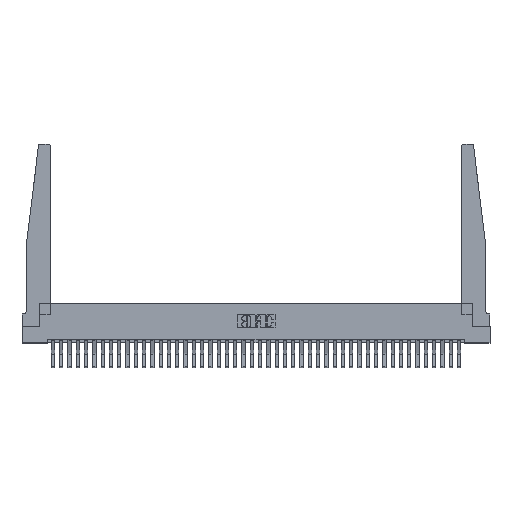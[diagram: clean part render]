
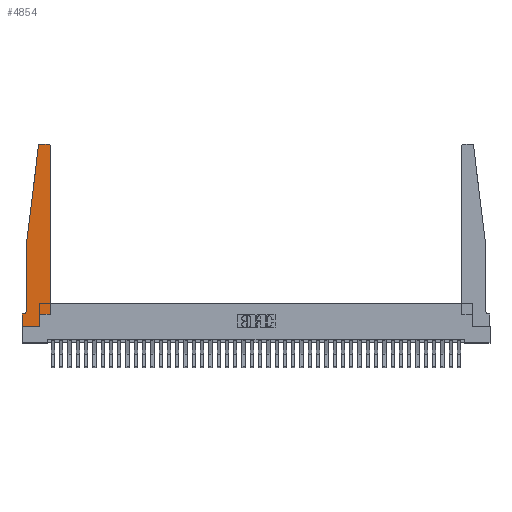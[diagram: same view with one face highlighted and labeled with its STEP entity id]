
A CAD part, top view. The second image highlights one B-rep face of the part: STEP entity #4854.
In plain terms, the highlighted planar face has unit normal (0, 0, 1).
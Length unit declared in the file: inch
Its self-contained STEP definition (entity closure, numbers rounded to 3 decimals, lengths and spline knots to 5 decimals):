
#469 = VERTEX_POINT ( 'NONE', #24913 ) ;
#730 = DIRECTION ( 'NONE',  ( 0., -1., 0. ) ) ;
#1406 = VECTOR ( 'NONE', #34349, 39.37008 ) ;
#1655 = DIRECTION ( 'NONE',  ( 0., 0., 1. ) ) ;
#2003 = EDGE_LOOP ( 'NONE', ( #2684, #4446, #31776, #13478, #16946, #12337, #13465, #21515, #30687, #9007, #33362, #3967 ) ) ;
#2256 = LINE ( 'NONE', #27699, #36144 ) ;
#2684 = ORIENTED_EDGE ( 'NONE', *, *, #27348, .T. ) ;
#2996 = VECTOR ( 'NONE', #10991, 39.37008 ) ;
#3223 = CARTESIAN_POINT ( 'NONE',  ( 0.065, 1.25, 0.37 ) ) ;
#3450 = CARTESIAN_POINT ( 'NONE',  ( 0.425, 0.18, 0.37 ) ) ;
#3483 = CARTESIAN_POINT ( 'NONE',  ( 0.425, 2.72, 0.37 ) ) ;
#3559 = VECTOR ( 'NONE', #11921, 39.37008 ) ;
#3967 = ORIENTED_EDGE ( 'NONE', *, *, #20323, .T. ) ;
#4028 = CARTESIAN_POINT ( 'NONE',  ( 0.395, 2.75, 0.37 ) ) ;
#4446 = ORIENTED_EDGE ( 'NONE', *, *, #19675, .T. ) ;
#4649 = AXIS2_PLACEMENT_3D ( 'NONE', #33127, #22322, #8237 ) ;
#4854 = ADVANCED_FACE ( 'NONE', ( #5731 ), #15746, .T. ) ;
#5681 = CARTESIAN_POINT ( 'NONE',  ( 0.2605, 0.18, 0.37 ) ) ;
#5731 = FACE_OUTER_BOUND ( 'NONE', #2003, .T. ) ;
#5926 = VERTEX_POINT ( 'NONE', #10606 ) ;
#6012 = AXIS2_PLACEMENT_3D ( 'NONE', #32309, #1655, #33043 ) ;
#6776 = VECTOR ( 'NONE', #17466, 39.37008 ) ;
#8115 = VECTOR ( 'NONE', #18488, 39.37008 ) ;
#8237 = DIRECTION ( 'NONE',  ( 1., 0., 0. ) ) ;
#8424 = CARTESIAN_POINT ( 'NONE',  ( 0.425, 0.18, 0.37 ) ) ;
#8470 = LINE ( 'NONE', #3223, #1406 ) ;
#9007 = ORIENTED_EDGE ( 'NONE', *, *, #31423, .T. ) ;
#10284 = DIRECTION ( 'NONE',  ( 1., 0., 0. ) ) ;
#10368 = DIRECTION ( 'NONE',  ( -0.122, -0.992, 0. ) ) ;
#10606 = CARTESIAN_POINT ( 'NONE',  ( 0., 0.1875, 0.37 ) ) ;
#10640 = CARTESIAN_POINT ( 'NONE',  ( 0.015, 0.1875, 0.37 ) ) ;
#10991 = DIRECTION ( 'NONE',  ( 0., 1., 0. ) ) ;
#11059 = LINE ( 'NONE', #29067, #3559 ) ;
#11267 = CIRCLE ( 'NONE', #6012, 0.03 ) ;
#11921 = DIRECTION ( 'NONE',  ( 0., 1., 0. ) ) ;
#12337 = ORIENTED_EDGE ( 'NONE', *, *, #21358, .T. ) ;
#12899 = VERTEX_POINT ( 'NONE', #5681 ) ;
#13136 = DIRECTION ( 'NONE',  ( 0., 0., 1. ) ) ;
#13337 = CARTESIAN_POINT ( 'NONE',  ( 0.065, 1.25, 0.37 ) ) ;
#13465 = ORIENTED_EDGE ( 'NONE', *, *, #36258, .T. ) ;
#13478 = ORIENTED_EDGE ( 'NONE', *, *, #14838, .T. ) ;
#14048 = CARTESIAN_POINT ( 'NONE',  ( 0.065, 0.1875, 0.37 ) ) ;
#14838 = EDGE_CURVE ( 'NONE', #36027, #19788, #8470, .T. ) ;
#15075 = LINE ( 'NONE', #13337, #19918 ) ;
#15208 = EDGE_CURVE ( 'NONE', #19788, #27316, #26507, .T. ) ;
#15484 = EDGE_CURVE ( 'NONE', #16502, #12899, #11059, .T. ) ;
#15746 = PLANE ( 'NONE',  #28295 ) ;
#16502 = VERTEX_POINT ( 'NONE', #19774 ) ;
#16516 = CARTESIAN_POINT ( 'NONE',  ( 0.015, 0.2375, 0.37 ) ) ;
#16946 = ORIENTED_EDGE ( 'NONE', *, *, #15208, .T. ) ;
#17116 = CARTESIAN_POINT ( 'NONE',  ( 0.065, 0.2375, 0.37 ) ) ;
#17466 = DIRECTION ( 'NONE',  ( -1., 0., 0. ) ) ;
#17596 = CARTESIAN_POINT ( 'NONE',  ( 0., 0., 0.37 ) ) ;
#17909 = CARTESIAN_POINT ( 'NONE',  ( 0., 0., 0.37 ) ) ;
#18488 = DIRECTION ( 'NONE',  ( 1., 0., 0. ) ) ;
#18975 = EDGE_CURVE ( 'NONE', #34360, #22185, #25064, .T. ) ;
#19044 = DIRECTION ( 'NONE',  ( -1., 0., 0. ) ) ;
#19110 = VERTEX_POINT ( 'NONE', #33644 ) ;
#19675 = EDGE_CURVE ( 'NONE', #19110, #31331, #32009, .T. ) ;
#19774 = CARTESIAN_POINT ( 'NONE',  ( 0.2605, 0., 0.37 ) ) ;
#19788 = VERTEX_POINT ( 'NONE', #17116 ) ;
#19918 = VECTOR ( 'NONE', #10368, 39.37008 ) ;
#20323 = EDGE_CURVE ( 'NONE', #22185, #35194, #11267, .T. ) ;
#20734 = VECTOR ( 'NONE', #26781, 39.37008 ) ;
#21358 = EDGE_CURVE ( 'NONE', #27316, #5926, #31042, .T. ) ;
#21515 = ORIENTED_EDGE ( 'NONE', *, *, #27843, .T. ) ;
#22185 = VERTEX_POINT ( 'NONE', #3483 ) ;
#22322 = DIRECTION ( 'NONE',  ( 0., 0., 1. ) ) ;
#24913 = CARTESIAN_POINT ( 'NONE',  ( 0., 0., 0.37 ) ) ;
#25037 = DIRECTION ( 'NONE',  ( 0., 0., -1. ) ) ;
#25064 = LINE ( 'NONE', #33419, #2996 ) ;
#26507 = CIRCLE ( 'NONE', #36132, 0.05 ) ;
#26781 = DIRECTION ( 'NONE',  ( 1., 0., 0. ) ) ;
#27316 = VERTEX_POINT ( 'NONE', #10640 ) ;
#27348 = EDGE_CURVE ( 'NONE', #35194, #19110, #2256, .T. ) ;
#27699 = CARTESIAN_POINT ( 'NONE',  ( 0.25, 2.75, 0.37 ) ) ;
#27843 = EDGE_CURVE ( 'NONE', #469, #16502, #35668, .T. ) ;
#28295 = AXIS2_PLACEMENT_3D ( 'NONE', #35500, #13136, #10284 ) ;
#28514 = CARTESIAN_POINT ( 'NONE',  ( 0.24675, 2.72367, 0.37 ) ) ;
#29067 = CARTESIAN_POINT ( 'NONE',  ( 0.2605, 0.18, 0.37 ) ) ;
#30687 = ORIENTED_EDGE ( 'NONE', *, *, #15484, .T. ) ;
#31042 = LINE ( 'NONE', #14048, #6776 ) ;
#31331 = VERTEX_POINT ( 'NONE', #28514 ) ;
#31423 = EDGE_CURVE ( 'NONE', #12899, #34360, #34109, .T. ) ;
#31776 = ORIENTED_EDGE ( 'NONE', *, *, #32940, .T. ) ;
#32009 = CIRCLE ( 'NONE', #4649, 0.03 ) ;
#32309 = CARTESIAN_POINT ( 'NONE',  ( 0.395, 2.72, 0.37 ) ) ;
#32940 = EDGE_CURVE ( 'NONE', #31331, #36027, #15075, .T. ) ;
#33043 = DIRECTION ( 'NONE',  ( 1., 0., 0. ) ) ;
#33127 = CARTESIAN_POINT ( 'NONE',  ( 0.27653, 2.72, 0.37 ) ) ;
#33246 = DIRECTION ( 'NONE',  ( -1., 0., 0. ) ) ;
#33362 = ORIENTED_EDGE ( 'NONE', *, *, #18975, .T. ) ;
#33419 = CARTESIAN_POINT ( 'NONE',  ( 0.425, 0.18, 0.37 ) ) ;
#33644 = CARTESIAN_POINT ( 'NONE',  ( 0.27653, 2.75, 0.37 ) ) ;
#34109 = LINE ( 'NONE', #3450, #8115 ) ;
#34186 = LINE ( 'NONE', #17596, #35958 ) ;
#34349 = DIRECTION ( 'NONE',  ( 0., -1., 0. ) ) ;
#34360 = VERTEX_POINT ( 'NONE', #8424 ) ;
#35194 = VERTEX_POINT ( 'NONE', #4028 ) ;
#35500 = CARTESIAN_POINT ( 'NONE',  ( 0., 0.1875, 0.37 ) ) ;
#35668 = LINE ( 'NONE', #17909, #20734 ) ;
#35681 = CARTESIAN_POINT ( 'NONE',  ( 0.065, 1.25, 0.37 ) ) ;
#35958 = VECTOR ( 'NONE', #730, 39.37008 ) ;
#36027 = VERTEX_POINT ( 'NONE', #35681 ) ;
#36132 = AXIS2_PLACEMENT_3D ( 'NONE', #16516, #25037, #33246 ) ;
#36144 = VECTOR ( 'NONE', #19044, 39.37008 ) ;
#36258 = EDGE_CURVE ( 'NONE', #5926, #469, #34186, .T. ) ;
